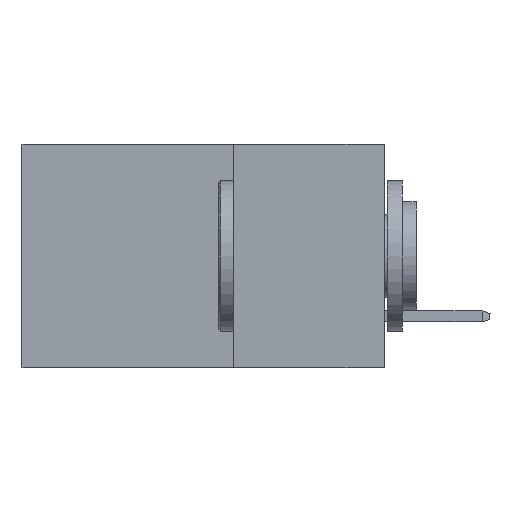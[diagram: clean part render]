
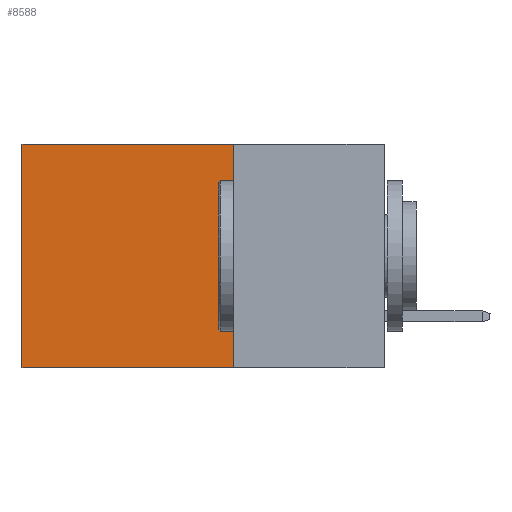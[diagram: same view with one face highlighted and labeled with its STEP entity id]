
A CAD part, left-side view. The second image highlights one B-rep face of the part: STEP entity #8588.
In plain terms, the highlighted planar face has unit normal (-1, 0, 0).
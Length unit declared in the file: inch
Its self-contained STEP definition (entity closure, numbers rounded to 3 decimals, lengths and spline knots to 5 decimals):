
#17 = VERTEX_POINT ( 'NONE', #3036 ) ;
#107 = EDGE_CURVE ( 'NONE', #8428, #17, #8692, .T. ) ;
#174 = ORIENTED_EDGE ( 'NONE', *, *, #10791, .T. ) ;
#221 = CARTESIAN_POINT ( 'NONE',  ( 0.2615, 0.6, -0.37 ) ) ;
#614 = CARTESIAN_POINT ( 'NONE',  ( 0.2615, 0.6, 0. ) ) ;
#640 = PLANE ( 'NONE',  #2063 ) ;
#1302 = DIRECTION ( 'NONE',  ( 1., 0., 0. ) ) ;
#1357 = FACE_OUTER_BOUND ( 'NONE', #4009, .T. ) ;
#1956 = DIRECTION ( 'NONE',  ( 0., 1., 0. ) ) ;
#2063 = AXIS2_PLACEMENT_3D ( 'NONE', #2310, #1302, #8303 ) ;
#2290 = VECTOR ( 'NONE', #2739, 39.37008 ) ;
#2310 = CARTESIAN_POINT ( 'NONE',  ( 0.2615, 0.25, -0.37 ) ) ;
#2554 = ORIENTED_EDGE ( 'NONE', *, *, #8317, .F. ) ;
#2586 = EDGE_CURVE ( 'NONE', #9460, #6991, #7366, .T. ) ;
#2739 = DIRECTION ( 'NONE',  ( 0., 0., -1. ) ) ;
#3006 = CARTESIAN_POINT ( 'NONE',  ( 0.2615, 0.25, 0. ) ) ;
#3033 = DIRECTION ( 'NONE',  ( 0., 0., -1. ) ) ;
#3036 = CARTESIAN_POINT ( 'NONE',  ( 0.2615, 0.25, -0.37 ) ) ;
#3996 = LINE ( 'NONE', #3006, #7729 ) ;
#4009 = EDGE_LOOP ( 'NONE', ( #6791, #2554, #7454, #174 ) ) ;
#4334 = LINE ( 'NONE', #8512, #9829 ) ;
#4812 = VECTOR ( 'NONE', #3033, 39.37008 ) ;
#5530 = CARTESIAN_POINT ( 'NONE',  ( 0.2615, 0.6, -0.37 ) ) ;
#6231 = CARTESIAN_POINT ( 'NONE',  ( 0.2615, 0.25, -0.37 ) ) ;
#6791 = ORIENTED_EDGE ( 'NONE', *, *, #2586, .T. ) ;
#6991 = VERTEX_POINT ( 'NONE', #221 ) ;
#7366 = LINE ( 'NONE', #5530, #4812 ) ;
#7454 = ORIENTED_EDGE ( 'NONE', *, *, #107, .F. ) ;
#7729 = VECTOR ( 'NONE', #8067, 39.37008 ) ;
#8067 = DIRECTION ( 'NONE',  ( 0., 1., 0. ) ) ;
#8122 = CARTESIAN_POINT ( 'NONE',  ( 0.2615, 0.25, 0. ) ) ;
#8303 = DIRECTION ( 'NONE',  ( 0., 0., -1. ) ) ;
#8317 = EDGE_CURVE ( 'NONE', #17, #6991, #4334, .T. ) ;
#8428 = VERTEX_POINT ( 'NONE', #8122 ) ;
#8512 = CARTESIAN_POINT ( 'NONE',  ( 0.2615, 0.25, -0.37 ) ) ;
#8588 = ADVANCED_FACE ( 'NONE', ( #1357 ), #640, .F. ) ;
#8692 = LINE ( 'NONE', #6231, #2290 ) ;
#9460 = VERTEX_POINT ( 'NONE', #614 ) ;
#9829 = VECTOR ( 'NONE', #1956, 39.37008 ) ;
#10791 = EDGE_CURVE ( 'NONE', #8428, #9460, #3996, .T. ) ;
